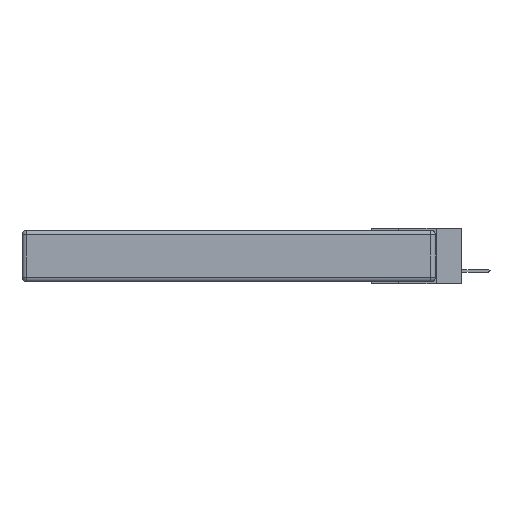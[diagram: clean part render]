
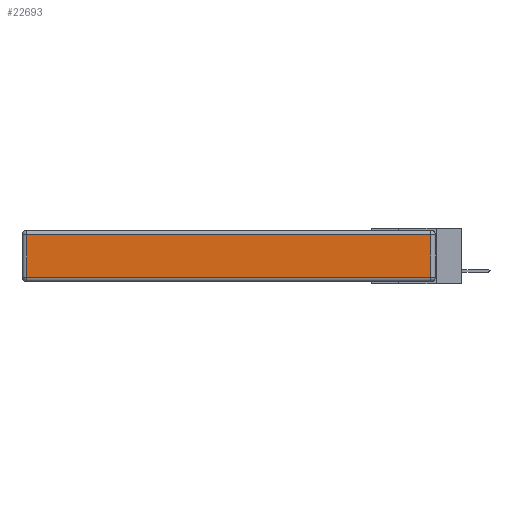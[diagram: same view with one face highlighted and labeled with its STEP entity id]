
A CAD part, left-side view. The second image highlights one B-rep face of the part: STEP entity #22693.
In plain terms, the highlighted planar face has unit normal (-1, 0, 0).
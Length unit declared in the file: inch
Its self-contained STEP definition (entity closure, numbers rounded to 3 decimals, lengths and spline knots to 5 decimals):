
#1040 = CARTESIAN_POINT ( 'NONE',  ( 0., 2.72, -0.03 ) ) ;
#1924 = CARTESIAN_POINT ( 'NONE',  ( 0., 2.72, -0.343 ) ) ;
#2287 = CARTESIAN_POINT ( 'NONE',  ( 0., 0.03, -0.03 ) ) ;
#2522 = DIRECTION ( 'NONE',  ( 0., -1., 0. ) ) ;
#3633 = VERTEX_POINT ( 'NONE', #2287 ) ;
#5821 = LINE ( 'NONE', #21645, #8197 ) ;
#6889 = PLANE ( 'NONE',  #17714 ) ;
#7054 = DIRECTION ( 'NONE',  ( 0., 0., 1. ) ) ;
#7632 = DIRECTION ( 'NONE',  ( 0., 0., -1. ) ) ;
#7937 = EDGE_LOOP ( 'NONE', ( #14637, #17849, #17168, #24754 ) ) ;
#8197 = VECTOR ( 'NONE', #2522, 39.37008 ) ;
#8472 = CARTESIAN_POINT ( 'NONE',  ( 0., 0.03, -0.313 ) ) ;
#9708 = EDGE_CURVE ( 'NONE', #11390, #10367, #5821, .T. ) ;
#10367 = VERTEX_POINT ( 'NONE', #8472 ) ;
#10962 = EDGE_CURVE ( 'NONE', #22849, #11390, #20611, .T. ) ;
#11390 = VERTEX_POINT ( 'NONE', #11611 ) ;
#11611 = CARTESIAN_POINT ( 'NONE',  ( 0., 2.72, -0.313 ) ) ;
#12025 = EDGE_CURVE ( 'NONE', #10367, #3633, #22358, .T. ) ;
#13180 = CARTESIAN_POINT ( 'NONE',  ( 0., 2.75, -0.03 ) ) ;
#13541 = VECTOR ( 'NONE', #21710, 39.37008 ) ;
#14637 = ORIENTED_EDGE ( 'NONE', *, *, #9708, .T. ) ;
#17168 = ORIENTED_EDGE ( 'NONE', *, *, #21304, .T. ) ;
#17296 = DIRECTION ( 'NONE',  ( 0., 1., 0. ) ) ;
#17714 = AXIS2_PLACEMENT_3D ( 'NONE', #18587, #24148, #7054 ) ;
#17849 = ORIENTED_EDGE ( 'NONE', *, *, #12025, .T. ) ;
#18587 = CARTESIAN_POINT ( 'NONE',  ( 0., 0., -0.343 ) ) ;
#19120 = FACE_OUTER_BOUND ( 'NONE', #7937, .T. ) ;
#19185 = VECTOR ( 'NONE', #17296, 39.37008 ) ;
#19393 = VECTOR ( 'NONE', #7632, 39.37008 ) ;
#20611 = LINE ( 'NONE', #1924, #19393 ) ;
#21304 = EDGE_CURVE ( 'NONE', #3633, #22849, #23696, .T. ) ;
#21645 = CARTESIAN_POINT ( 'NONE',  ( 0., 0., -0.313 ) ) ;
#21710 = DIRECTION ( 'NONE',  ( 0., 0., 1. ) ) ;
#22358 = LINE ( 'NONE', #23560, #13541 ) ;
#22693 = ADVANCED_FACE ( 'NONE', ( #19120 ), #6889, .T. ) ;
#22849 = VERTEX_POINT ( 'NONE', #1040 ) ;
#23560 = CARTESIAN_POINT ( 'NONE',  ( 0., 0.03, -0.343 ) ) ;
#23696 = LINE ( 'NONE', #13180, #19185 ) ;
#24148 = DIRECTION ( 'NONE',  ( -1., 0., 0. ) ) ;
#24754 = ORIENTED_EDGE ( 'NONE', *, *, #10962, .T. ) ;
